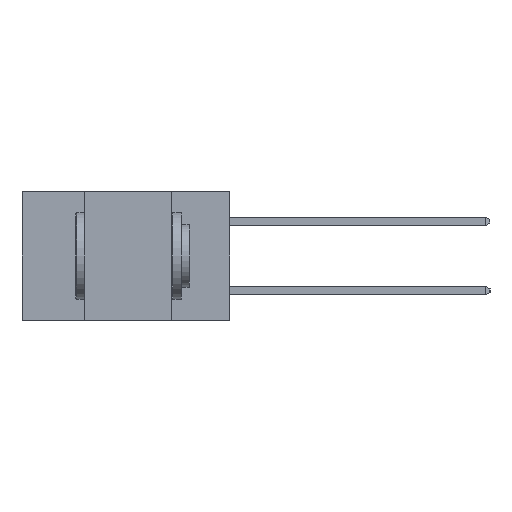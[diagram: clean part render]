
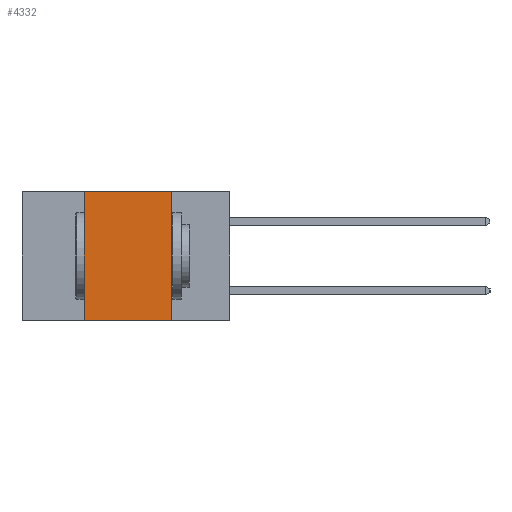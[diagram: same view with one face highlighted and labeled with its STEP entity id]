
A CAD part, left-side view. The second image highlights one B-rep face of the part: STEP entity #4332.
In plain terms, the highlighted planar face has unit normal (-1, 0, 0).
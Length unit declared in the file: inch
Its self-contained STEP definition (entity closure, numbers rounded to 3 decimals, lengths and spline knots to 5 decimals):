
#81 = FACE_OUTER_BOUND ( 'NONE', #4452, .T. ) ;
#666 = VECTOR ( 'NONE', #5468, 39.37008 ) ;
#1397 = VECTOR ( 'NONE', #9991, 39.37008 ) ;
#1653 = ORIENTED_EDGE ( 'NONE', *, *, #1924, .F. ) ;
#1760 = LINE ( 'NONE', #9915, #1397 ) ;
#1893 = CARTESIAN_POINT ( 'NONE',  ( 0., 0.42, 0. ) ) ;
#1924 = EDGE_CURVE ( 'NONE', #3624, #14495, #10202, .T. ) ;
#2498 = LINE ( 'NONE', #14447, #2905 ) ;
#2760 = EDGE_CURVE ( 'NONE', #3624, #6875, #8884, .T. ) ;
#2905 = VECTOR ( 'NONE', #14448, 39.37008 ) ;
#2997 = ORIENTED_EDGE ( 'NONE', *, *, #12743, .F. ) ;
#3624 = VERTEX_POINT ( 'NONE', #11976 ) ;
#4190 = CARTESIAN_POINT ( 'NONE',  ( 0., 0.17, 0. ) ) ;
#4332 = ADVANCED_FACE ( 'NONE', ( #81 ), #13585, .F. ) ;
#4452 = EDGE_LOOP ( 'NONE', ( #10264, #2997, #1653, #13549 ) ) ;
#5468 = DIRECTION ( 'NONE',  ( 0., 0., 1. ) ) ;
#5501 = CARTESIAN_POINT ( 'NONE',  ( 0., 0.42, -0.37 ) ) ;
#6000 = CARTESIAN_POINT ( 'NONE',  ( 0., 0.6, -0.37 ) ) ;
#6161 = DIRECTION ( 'NONE',  ( 0., -1., 0. ) ) ;
#6875 = VERTEX_POINT ( 'NONE', #9014 ) ;
#8884 = LINE ( 'NONE', #6000, #11651 ) ;
#9014 = CARTESIAN_POINT ( 'NONE',  ( 0., 0.17, -0.37 ) ) ;
#9413 = AXIS2_PLACEMENT_3D ( 'NONE', #12795, #12793, #12742 ) ;
#9915 = CARTESIAN_POINT ( 'NONE',  ( 0., 0.17, -0.37 ) ) ;
#9991 = DIRECTION ( 'NONE',  ( 0., 0., -1. ) ) ;
#10202 = LINE ( 'NONE', #5501, #666 ) ;
#10264 = ORIENTED_EDGE ( 'NONE', *, *, #13460, .F. ) ;
#11044 = VERTEX_POINT ( 'NONE', #4190 ) ;
#11651 = VECTOR ( 'NONE', #6161, 39.37008 ) ;
#11976 = CARTESIAN_POINT ( 'NONE',  ( 0., 0.42, -0.37 ) ) ;
#12742 = DIRECTION ( 'NONE',  ( 0., 0., -1. ) ) ;
#12743 = EDGE_CURVE ( 'NONE', #14495, #11044, #2498, .T. ) ;
#12793 = DIRECTION ( 'NONE',  ( 1., 0., 0. ) ) ;
#12795 = CARTESIAN_POINT ( 'NONE',  ( 0., 0.6, 0. ) ) ;
#13460 = EDGE_CURVE ( 'NONE', #11044, #6875, #1760, .T. ) ;
#13549 = ORIENTED_EDGE ( 'NONE', *, *, #2760, .T. ) ;
#13585 = PLANE ( 'NONE',  #9413 ) ;
#14447 = CARTESIAN_POINT ( 'NONE',  ( 0., 0.6, 0. ) ) ;
#14448 = DIRECTION ( 'NONE',  ( 0., -1., 0. ) ) ;
#14495 = VERTEX_POINT ( 'NONE', #1893 ) ;
